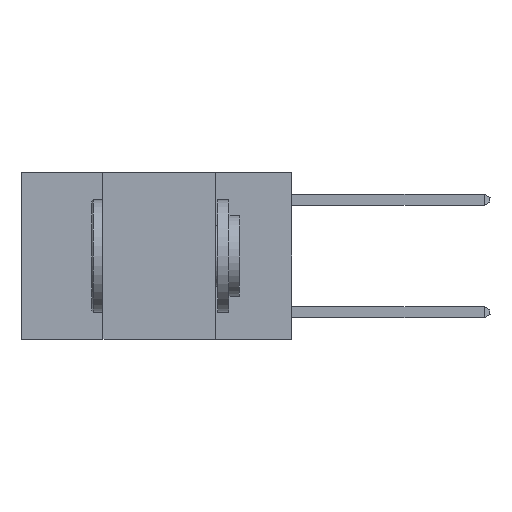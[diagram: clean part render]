
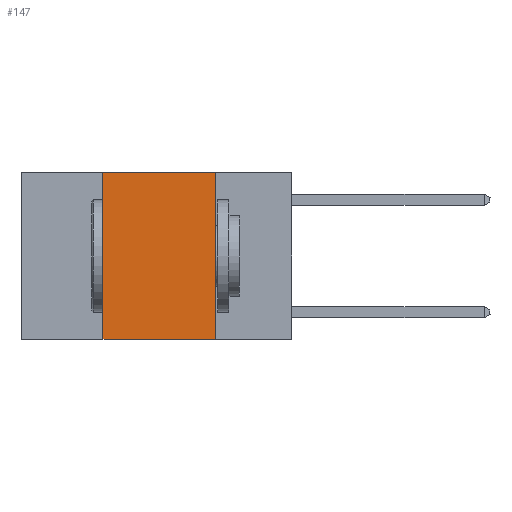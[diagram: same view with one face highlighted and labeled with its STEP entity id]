
A CAD part, left-side view. The second image highlights one B-rep face of the part: STEP entity #147.
In plain terms, the highlighted planar face has unit normal (-1, 0, 0).
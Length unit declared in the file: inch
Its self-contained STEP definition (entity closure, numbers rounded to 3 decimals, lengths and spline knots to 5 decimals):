
#147 = ADVANCED_FACE ( 'NONE', ( #19820 ), #12191, .F. ) ;
#2883 = DIRECTION ( 'NONE',  ( 0., 0., 1. ) ) ;
#3117 = LINE ( 'NONE', #6609, #24439 ) ;
#3249 = DIRECTION ( 'NONE',  ( 0., -1., 0. ) ) ;
#4254 = CARTESIAN_POINT ( 'NONE',  ( 0., 0.6, 0. ) ) ;
#4573 = LINE ( 'NONE', #4823, #7288 ) ;
#4823 = CARTESIAN_POINT ( 'NONE',  ( 0., 0.42, 0. ) ) ;
#5181 = EDGE_CURVE ( 'NONE', #21393, #6962, #4573, .T. ) ;
#5318 = CARTESIAN_POINT ( 'NONE',  ( 0., 0.42, 0. ) ) ;
#5592 = CARTESIAN_POINT ( 'NONE',  ( 0., 0.17, 0. ) ) ;
#6609 = CARTESIAN_POINT ( 'NONE',  ( 0., 0.6, -0.37 ) ) ;
#6962 = VERTEX_POINT ( 'NONE', #5318 ) ;
#7288 = VECTOR ( 'NONE', #2883, 39.37008 ) ;
#7680 = VECTOR ( 'NONE', #23913, 39.37008 ) ;
#7956 = DIRECTION ( 'NONE',  ( 1., 0., 0. ) ) ;
#10085 = EDGE_CURVE ( 'NONE', #6962, #19398, #18016, .T. ) ;
#10950 = CARTESIAN_POINT ( 'NONE',  ( 0., 0.17, 0. ) ) ;
#12191 = PLANE ( 'NONE',  #21967 ) ;
#12779 = EDGE_CURVE ( 'NONE', #21393, #15514, #3117, .T. ) ;
#14562 = DIRECTION ( 'NONE',  ( 0., 0., -1. ) ) ;
#14865 = EDGE_CURVE ( 'NONE', #19398, #15514, #25394, .T. ) ;
#15514 = VERTEX_POINT ( 'NONE', #21441 ) ;
#17376 = CARTESIAN_POINT ( 'NONE',  ( 0., 0.42, -0.37 ) ) ;
#17761 = ORIENTED_EDGE ( 'NONE', *, *, #10085, .F. ) ;
#17802 = VECTOR ( 'NONE', #19122, 39.37008 ) ;
#18016 = LINE ( 'NONE', #4254, #7680 ) ;
#19122 = DIRECTION ( 'NONE',  ( 0., 0., -1. ) ) ;
#19398 = VERTEX_POINT ( 'NONE', #10950 ) ;
#19820 = FACE_OUTER_BOUND ( 'NONE', #20095, .T. ) ;
#20086 = CARTESIAN_POINT ( 'NONE',  ( 0., 0.6, 0. ) ) ;
#20095 = EDGE_LOOP ( 'NONE', ( #21863, #17761, #21520, #22751 ) ) ;
#21393 = VERTEX_POINT ( 'NONE', #17376 ) ;
#21441 = CARTESIAN_POINT ( 'NONE',  ( 0., 0.17, -0.37 ) ) ;
#21520 = ORIENTED_EDGE ( 'NONE', *, *, #5181, .F. ) ;
#21863 = ORIENTED_EDGE ( 'NONE', *, *, #14865, .F. ) ;
#21967 = AXIS2_PLACEMENT_3D ( 'NONE', #20086, #7956, #14562 ) ;
#22751 = ORIENTED_EDGE ( 'NONE', *, *, #12779, .T. ) ;
#23913 = DIRECTION ( 'NONE',  ( 0., -1., 0. ) ) ;
#24439 = VECTOR ( 'NONE', #3249, 39.37008 ) ;
#25394 = LINE ( 'NONE', #5592, #17802 ) ;
